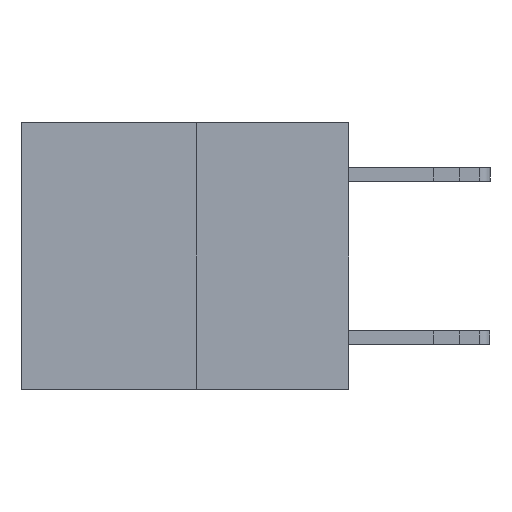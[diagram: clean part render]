
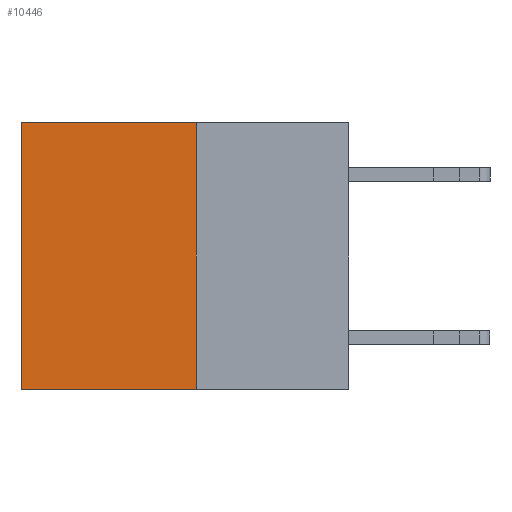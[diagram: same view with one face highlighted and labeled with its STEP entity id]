
A CAD part, left-side view. The second image highlights one B-rep face of the part: STEP entity #10446.
In plain terms, the highlighted planar face has unit normal (-1, 0, 0).
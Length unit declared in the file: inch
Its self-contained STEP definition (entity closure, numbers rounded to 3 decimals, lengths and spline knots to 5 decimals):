
#457 = DIRECTION ( 'NONE',  ( 0., 0., -1. ) ) ;
#1094 = LINE ( 'NONE', #4089, #10552 ) ;
#3014 = DIRECTION ( 'NONE',  ( 0., 1., 0. ) ) ;
#3038 = LINE ( 'NONE', #7003, #17212 ) ;
#3219 = PLANE ( 'NONE',  #12408 ) ;
#3448 = CARTESIAN_POINT ( 'NONE',  ( 0.3165, 0.28, -0.49 ) ) ;
#3625 = FACE_OUTER_BOUND ( 'NONE', #12654, .T. ) ;
#4064 = EDGE_CURVE ( 'NONE', #9285, #4143, #3038, .T. ) ;
#4067 = ORIENTED_EDGE ( 'NONE', *, *, #4064, .T. ) ;
#4089 = CARTESIAN_POINT ( 'NONE',  ( 0.3165, 0.28, -0.49 ) ) ;
#4143 = VERTEX_POINT ( 'NONE', #12416 ) ;
#4765 = EDGE_CURVE ( 'NONE', #9859, #4143, #1094, .T. ) ;
#5430 = DIRECTION ( 'NONE',  ( 0., 1., 0. ) ) ;
#5741 = CARTESIAN_POINT ( 'NONE',  ( 0.3165, 0.28, -0.49 ) ) ;
#6432 = LINE ( 'NONE', #6804, #14305 ) ;
#6675 = VECTOR ( 'NONE', #457, 39.37008 ) ;
#6804 = CARTESIAN_POINT ( 'NONE',  ( 0.3165, 0.28, 0. ) ) ;
#7003 = CARTESIAN_POINT ( 'NONE',  ( 0.3165, 0.6, -0.49 ) ) ;
#8177 = ORIENTED_EDGE ( 'NONE', *, *, #9742, .F. ) ;
#8413 = ORIENTED_EDGE ( 'NONE', *, *, #4765, .F. ) ;
#9285 = VERTEX_POINT ( 'NONE', #11988 ) ;
#9742 = EDGE_CURVE ( 'NONE', #14990, #9859, #10147, .T. ) ;
#9859 = VERTEX_POINT ( 'NONE', #3448 ) ;
#10147 = LINE ( 'NONE', #11201, #6675 ) ;
#10446 = ADVANCED_FACE ( 'NONE', ( #3625 ), #3219, .F. ) ;
#10552 = VECTOR ( 'NONE', #3014, 39.37008 ) ;
#11201 = CARTESIAN_POINT ( 'NONE',  ( 0.3165, 0.28, -0.49 ) ) ;
#11880 = CARTESIAN_POINT ( 'NONE',  ( 0.3165, 0.28, 0. ) ) ;
#11988 = CARTESIAN_POINT ( 'NONE',  ( 0.3165, 0.6, 0. ) ) ;
#12408 = AXIS2_PLACEMENT_3D ( 'NONE', #5741, #16910, #15465 ) ;
#12416 = CARTESIAN_POINT ( 'NONE',  ( 0.3165, 0.6, -0.49 ) ) ;
#12654 = EDGE_LOOP ( 'NONE', ( #4067, #8413, #8177, #14597 ) ) ;
#12861 = EDGE_CURVE ( 'NONE', #14990, #9285, #6432, .T. ) ;
#13802 = DIRECTION ( 'NONE',  ( 0., 0., -1. ) ) ;
#14305 = VECTOR ( 'NONE', #5430, 39.37008 ) ;
#14597 = ORIENTED_EDGE ( 'NONE', *, *, #12861, .T. ) ;
#14990 = VERTEX_POINT ( 'NONE', #11880 ) ;
#15465 = DIRECTION ( 'NONE',  ( 0., 0., -1. ) ) ;
#16910 = DIRECTION ( 'NONE',  ( 1., 0., 0. ) ) ;
#17212 = VECTOR ( 'NONE', #13802, 39.37008 ) ;
